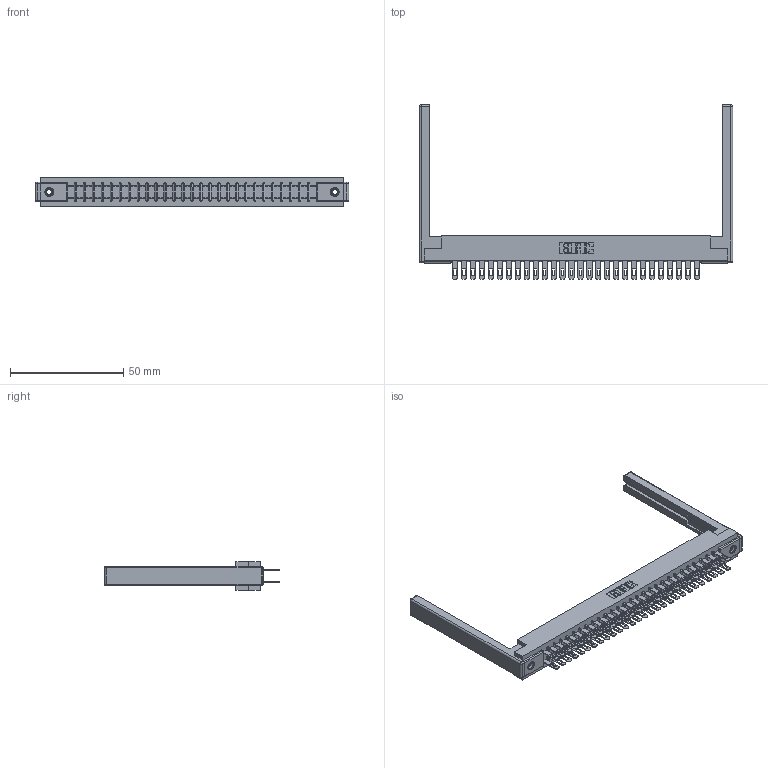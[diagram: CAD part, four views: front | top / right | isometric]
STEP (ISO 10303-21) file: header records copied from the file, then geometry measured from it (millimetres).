
FILE_DESCRIPTION (( 'STEP AP203' ), '1' );
FILE_NAME ('357-056-500-268.STEP', '2019-09-19T04:27:40', ( '' ), ( '' ), 'SwSTEP 2.0', 'SolidWorks 2016', '' );
FILE_SCHEMA (( 'CONFIG_CONTROL_DESIGN' ));
Length unit declared in the file: inch
Products named in the file (5): 307 Part_.156 Dia Mounting Holes; 357-056-500-268; 345-250-001_345-250-001-102; 307-290-001_500; 307-220-068
Assembly tree (61 placements, depth 2):
  357-056-500-268
    307 Part_.156 Dia Mounting Holes
    307-290-001_500  x56
    307-220-068  x2
    345-250-001_345-250-001-102  x2
Bounding box: 138.38 x 77.14 x 12.7 mm (x, y, z)
Volume: 19156.8 mm3; surface area: 22670.2 mm2
Topology: 61 solids, 61 shells, 2877 faces, 7993 edges, 5154 vertices
Faces by surface type: plane 1838, cylinder 957, sphere 66, cone 12, torus 4
Entity records: 29359 total; most frequent: CARTESIAN_POINT 4781, ORIENTED_EDGE 4728, DIRECTION 4706, EDGE_CURVE 2364, LINE 1804, VECTOR 1804, VERTEX_POINT 1526, AXIS2_PLACEMENT_3D 1451
